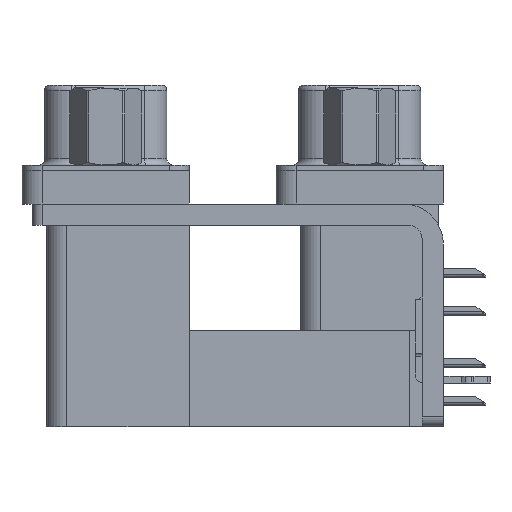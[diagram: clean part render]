
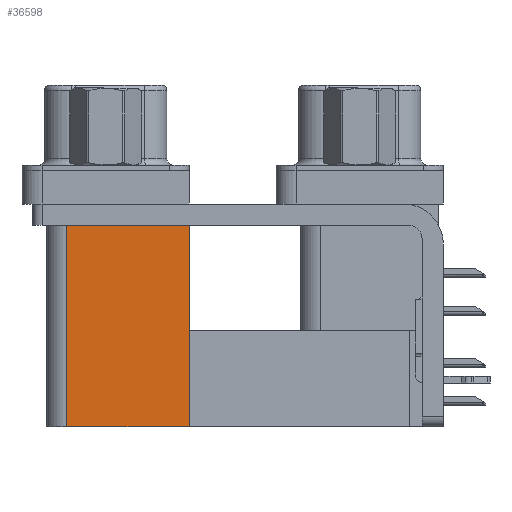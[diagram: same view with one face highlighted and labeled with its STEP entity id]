
A CAD part, left-side view. The second image highlights one B-rep face of the part: STEP entity #36598.
In plain terms, the highlighted planar face has unit normal (-1, 0, 0).
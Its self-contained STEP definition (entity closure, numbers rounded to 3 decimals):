
#814 = AXIS2_PLACEMENT_3D ( 'NONE', #14172, #13978, #22837 ) ;
#1397 = VERTEX_POINT ( 'NONE', #26716 ) ;
#4098 = LINE ( 'NONE', #24328, #14744 ) ;
#4369 = EDGE_CURVE ( 'NONE', #16466, #1397, #28372, .T. ) ;
#6291 = CARTESIAN_POINT ( 'NONE',  ( 3.765, 12.775, -19.2 ) ) ;
#8791 = FACE_OUTER_BOUND ( 'NONE', #16302, .T. ) ;
#10121 = ORIENTED_EDGE ( 'NONE', *, *, #15742, .F. ) ;
#10311 = EDGE_CURVE ( 'NONE', #36750, #16466, #36865, .T. ) ;
#10640 = CARTESIAN_POINT ( 'NONE',  ( 3.765, 12.775, -19.2 ) ) ;
#11423 = CARTESIAN_POINT ( 'NONE',  ( 3.765, 12.775, -2.5 ) ) ;
#12105 = ORIENTED_EDGE ( 'NONE', *, *, #20747, .F. ) ;
#12758 = DIRECTION ( 'NONE',  ( 0., 1., 0. ) ) ;
#13323 = VECTOR ( 'NONE', #15859, 1000. ) ;
#13978 = DIRECTION ( 'NONE',  ( 1., 0., 0. ) ) ;
#14172 = CARTESIAN_POINT ( 'NONE',  ( 3.765, 12.775, -19.2 ) ) ;
#14744 = VECTOR ( 'NONE', #12758, 1000. ) ;
#15742 = EDGE_CURVE ( 'NONE', #30343, #1397, #27543, .T. ) ;
#15859 = DIRECTION ( 'NONE',  ( 0., 0., 1. ) ) ;
#16302 = EDGE_LOOP ( 'NONE', ( #37911, #10121, #12105, #36704 ) ) ;
#16466 = VERTEX_POINT ( 'NONE', #17079 ) ;
#17079 = CARTESIAN_POINT ( 'NONE',  ( 3.765, 12.775, -2.5 ) ) ;
#17402 = DIRECTION ( 'NONE',  ( 0., 1., 0. ) ) ;
#19020 = VECTOR ( 'NONE', #36432, 1000. ) ;
#20747 = EDGE_CURVE ( 'NONE', #36750, #30343, #4098, .T. ) ;
#22837 = DIRECTION ( 'NONE',  ( 0., 0., -1. ) ) ;
#23568 = VECTOR ( 'NONE', #17402, 1000. ) ;
#24289 = CARTESIAN_POINT ( 'NONE',  ( 3.765, 21.975, -19.2 ) ) ;
#24328 = CARTESIAN_POINT ( 'NONE',  ( 3.765, 12.775, -19.2 ) ) ;
#26716 = CARTESIAN_POINT ( 'NONE',  ( 3.765, 21.975, -2.5 ) ) ;
#27543 = LINE ( 'NONE', #24289, #19020 ) ;
#28372 = LINE ( 'NONE', #11423, #23568 ) ;
#29012 = PLANE ( 'NONE',  #814 ) ;
#30343 = VERTEX_POINT ( 'NONE', #30356 ) ;
#30356 = CARTESIAN_POINT ( 'NONE',  ( 3.765, 21.975, -19.2 ) ) ;
#36432 = DIRECTION ( 'NONE',  ( 0., 0., 1. ) ) ;
#36598 = ADVANCED_FACE ( 'NONE', ( #8791 ), #29012, .F. ) ;
#36704 = ORIENTED_EDGE ( 'NONE', *, *, #10311, .T. ) ;
#36750 = VERTEX_POINT ( 'NONE', #6291 ) ;
#36865 = LINE ( 'NONE', #10640, #13323 ) ;
#37911 = ORIENTED_EDGE ( 'NONE', *, *, #4369, .T. ) ;
